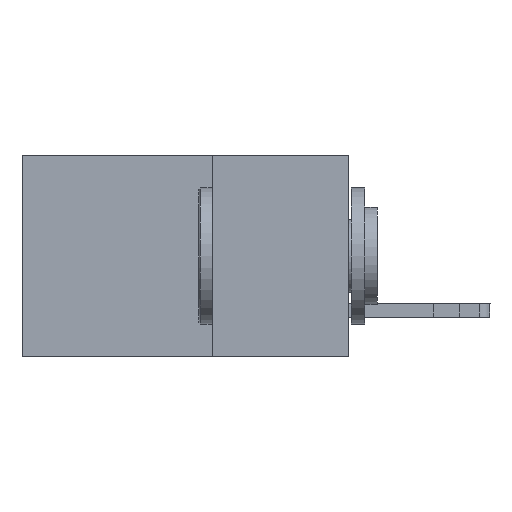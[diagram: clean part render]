
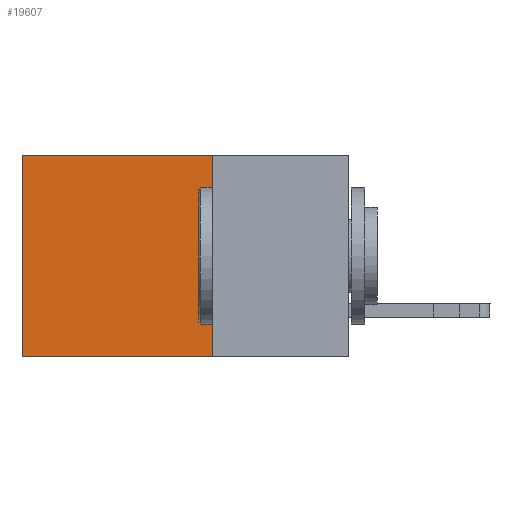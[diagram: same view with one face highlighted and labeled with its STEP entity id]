
A CAD part, left-side view. The second image highlights one B-rep face of the part: STEP entity #19607.
In plain terms, the highlighted planar face has unit normal (-1, 0, 0).
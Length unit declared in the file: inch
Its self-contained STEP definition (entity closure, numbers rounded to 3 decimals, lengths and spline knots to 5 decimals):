
#2440 = CARTESIAN_POINT ( 'NONE',  ( 0.2615, 0.6, 0. ) ) ;
#2577 = EDGE_LOOP ( 'NONE', ( #16616, #13230, #18176, #10287 ) ) ;
#2902 = LINE ( 'NONE', #4484, #12186 ) ;
#3174 = DIRECTION ( 'NONE',  ( 0., 0., -1. ) ) ;
#3195 = CARTESIAN_POINT ( 'NONE',  ( 0.2615, 0.25, -0.37 ) ) ;
#3247 = DIRECTION ( 'NONE',  ( 0., 0., -1. ) ) ;
#3780 = EDGE_CURVE ( 'NONE', #7321, #16990, #2902, .T. ) ;
#4188 = VECTOR ( 'NONE', #12997, 39.37008 ) ;
#4479 = DIRECTION ( 'NONE',  ( 0., 1., 0. ) ) ;
#4484 = CARTESIAN_POINT ( 'NONE',  ( 0.2615, 0.25, 0. ) ) ;
#4701 = EDGE_CURVE ( 'NONE', #19615, #19000, #8182, .T. ) ;
#7296 = LINE ( 'NONE', #17547, #4188 ) ;
#7321 = VERTEX_POINT ( 'NONE', #9804 ) ;
#7693 = VECTOR ( 'NONE', #12828, 39.37008 ) ;
#8182 = LINE ( 'NONE', #12438, #7693 ) ;
#9402 = CARTESIAN_POINT ( 'NONE',  ( 0.2615, 0.25, -0.37 ) ) ;
#9804 = CARTESIAN_POINT ( 'NONE',  ( 0.2615, 0.25, 0. ) ) ;
#10287 = ORIENTED_EDGE ( 'NONE', *, *, #3780, .T. ) ;
#10926 = CARTESIAN_POINT ( 'NONE',  ( 0.2615, 0.25, -0.37 ) ) ;
#11150 = CARTESIAN_POINT ( 'NONE',  ( 0.2615, 0.6, -0.37 ) ) ;
#11211 = EDGE_CURVE ( 'NONE', #16990, #19000, #7296, .T. ) ;
#11416 = VECTOR ( 'NONE', #3247, 39.37008 ) ;
#12186 = VECTOR ( 'NONE', #4479, 39.37008 ) ;
#12438 = CARTESIAN_POINT ( 'NONE',  ( 0.2615, 0.25, -0.37 ) ) ;
#12507 = DIRECTION ( 'NONE',  ( 1., 0., 0. ) ) ;
#12828 = DIRECTION ( 'NONE',  ( 0., 1., 0. ) ) ;
#12997 = DIRECTION ( 'NONE',  ( 0., 0., -1. ) ) ;
#13230 = ORIENTED_EDGE ( 'NONE', *, *, #4701, .F. ) ;
#13539 = AXIS2_PLACEMENT_3D ( 'NONE', #10926, #12507, #3174 ) ;
#14631 = FACE_OUTER_BOUND ( 'NONE', #2577, .T. ) ;
#16616 = ORIENTED_EDGE ( 'NONE', *, *, #11211, .T. ) ;
#16990 = VERTEX_POINT ( 'NONE', #2440 ) ;
#17547 = CARTESIAN_POINT ( 'NONE',  ( 0.2615, 0.6, -0.37 ) ) ;
#17781 = EDGE_CURVE ( 'NONE', #7321, #19615, #19478, .T. ) ;
#18176 = ORIENTED_EDGE ( 'NONE', *, *, #17781, .F. ) ;
#19000 = VERTEX_POINT ( 'NONE', #11150 ) ;
#19478 = LINE ( 'NONE', #3195, #11416 ) ;
#19607 = ADVANCED_FACE ( 'NONE', ( #14631 ), #20011, .F. ) ;
#19615 = VERTEX_POINT ( 'NONE', #9402 ) ;
#20011 = PLANE ( 'NONE',  #13539 ) ;
